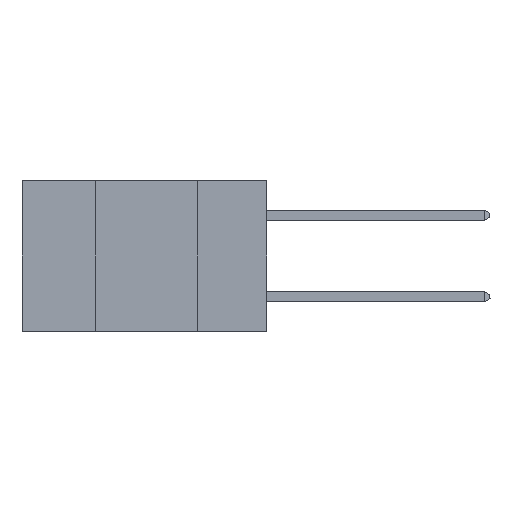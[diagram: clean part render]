
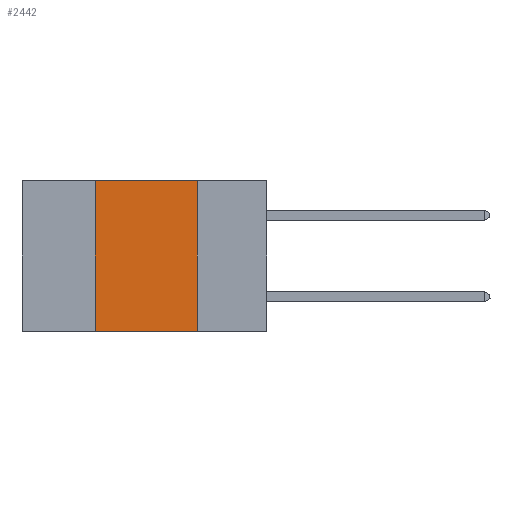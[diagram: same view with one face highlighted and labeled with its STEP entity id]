
A CAD part, left-side view. The second image highlights one B-rep face of the part: STEP entity #2442.
In plain terms, the highlighted planar face has unit normal (-1, 0, 0).
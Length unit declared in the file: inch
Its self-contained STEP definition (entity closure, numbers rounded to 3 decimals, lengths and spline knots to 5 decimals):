
#2442 = ADVANCED_FACE ( 'NONE', ( #22691 ), #30797, .F. ) ;
#3591 = EDGE_CURVE ( 'NONE', #12343, #12957, #28226, .T. ) ;
#5428 = DIRECTION ( 'NONE',  ( 0., 0., -1. ) ) ;
#5813 = VECTOR ( 'NONE', #32234, 39.37008 ) ;
#6950 = CARTESIAN_POINT ( 'NONE',  ( 0., 0.42, -0.37 ) ) ;
#7067 = CARTESIAN_POINT ( 'NONE',  ( 0., 0.42, 0. ) ) ;
#7548 = LINE ( 'NONE', #41432, #26031 ) ;
#9495 = CARTESIAN_POINT ( 'NONE',  ( 0., 0.6, 0. ) ) ;
#12343 = VERTEX_POINT ( 'NONE', #6950 ) ;
#12957 = VERTEX_POINT ( 'NONE', #18289 ) ;
#13196 = CARTESIAN_POINT ( 'NONE',  ( 0., 0.6, 0. ) ) ;
#13668 = DIRECTION ( 'NONE',  ( 0., -1., 0. ) ) ;
#14766 = VECTOR ( 'NONE', #13668, 39.37008 ) ;
#15087 = EDGE_CURVE ( 'NONE', #16531, #37193, #7548, .T. ) ;
#15774 = DIRECTION ( 'NONE',  ( 0., -1., 0. ) ) ;
#16531 = VERTEX_POINT ( 'NONE', #17462 ) ;
#16913 = DIRECTION ( 'NONE',  ( 1., 0., 0. ) ) ;
#17462 = CARTESIAN_POINT ( 'NONE',  ( 0., 0.17, 0. ) ) ;
#18289 = CARTESIAN_POINT ( 'NONE',  ( 0., 0.42, 0. ) ) ;
#20765 = CARTESIAN_POINT ( 'NONE',  ( 0., 0.17, -0.37 ) ) ;
#21704 = VECTOR ( 'NONE', #15774, 39.37008 ) ;
#22369 = ORIENTED_EDGE ( 'NONE', *, *, #22864, .F. ) ;
#22691 = FACE_OUTER_BOUND ( 'NONE', #41447, .T. ) ;
#22864 = EDGE_CURVE ( 'NONE', #12957, #16531, #42317, .T. ) ;
#26031 = VECTOR ( 'NONE', #5428, 39.37008 ) ;
#28002 = AXIS2_PLACEMENT_3D ( 'NONE', #9495, #16913, #41499 ) ;
#28226 = LINE ( 'NONE', #7067, #5813 ) ;
#28729 = ORIENTED_EDGE ( 'NONE', *, *, #3591, .F. ) ;
#30797 = PLANE ( 'NONE',  #28002 ) ;
#32234 = DIRECTION ( 'NONE',  ( 0., 0., 1. ) ) ;
#32284 = EDGE_CURVE ( 'NONE', #12343, #37193, #36136, .T. ) ;
#33378 = CARTESIAN_POINT ( 'NONE',  ( 0., 0.6, -0.37 ) ) ;
#34907 = ORIENTED_EDGE ( 'NONE', *, *, #15087, .F. ) ;
#36136 = LINE ( 'NONE', #33378, #21704 ) ;
#37193 = VERTEX_POINT ( 'NONE', #20765 ) ;
#41432 = CARTESIAN_POINT ( 'NONE',  ( 0., 0.17, 0. ) ) ;
#41447 = EDGE_LOOP ( 'NONE', ( #34907, #22369, #28729, #43868 ) ) ;
#41499 = DIRECTION ( 'NONE',  ( 0., 0., -1. ) ) ;
#42317 = LINE ( 'NONE', #13196, #14766 ) ;
#43868 = ORIENTED_EDGE ( 'NONE', *, *, #32284, .T. ) ;
